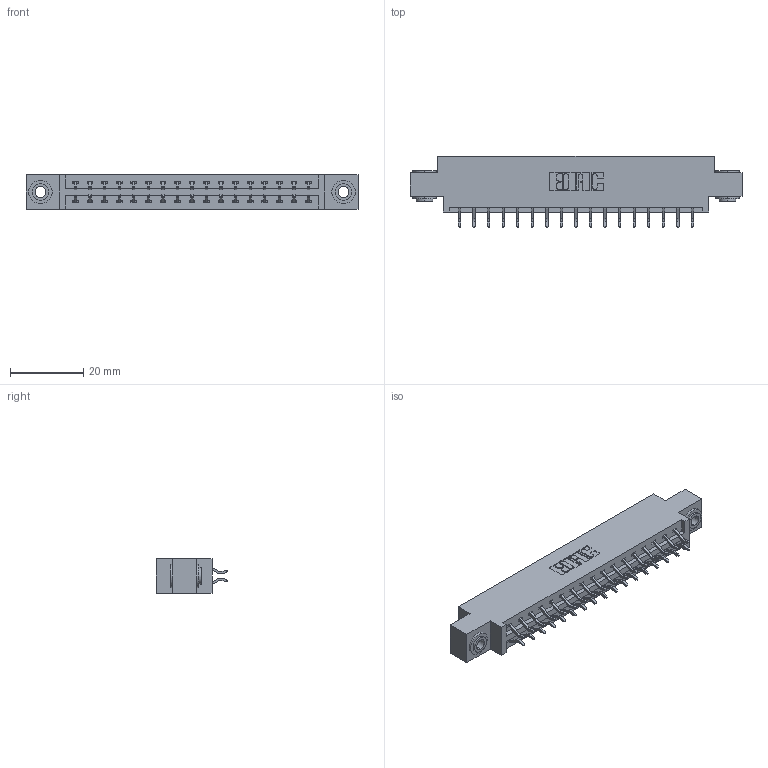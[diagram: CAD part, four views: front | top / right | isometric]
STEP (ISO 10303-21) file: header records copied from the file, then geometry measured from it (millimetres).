
FILE_DESCRIPTION (( 'STEP AP203' ), '1' );
FILE_NAME ('337-034-556-803.STEP', '2018-08-07T13:22:19', ( '' ), ( '' ), 'SwSTEP 2.0', 'SolidWorks 2016', '' );
FILE_SCHEMA (( 'CONFIG_CONTROL_DESIGN' ));
Length unit declared in the file: inch
Products named in the file (4): 345-292-001_556 Tail; 345-250-002_345-250-002-102; 337-034-556-803; 337 Part_0.170 Offset - 0.156 Dia-TH
Assembly tree (37 placements, depth 2):
  337-034-556-803
    337 Part_0.170 Offset - 0.156 Dia-TH
    345-292-001_556 Tail  x34
    345-250-002_345-250-002-102  x2
Bounding box: 90.37 x 19.57 x 9.4 mm (x, y, z)
Volume: 9092 mm3; surface area: 10332.1 mm2
Topology: 37 solids, 37 shells, 2196 faces, 6485 edges, 4274 vertices
Faces by surface type: plane 1512, cylinder 676, cone 8
Entity records: 17416 total; most frequent: CARTESIAN_POINT 2945, ORIENTED_EDGE 2862, DIRECTION 2573, EDGE_CURVE 1431, VECTOR 1271, LINE 1271, VERTEX_POINT 950, AXIS2_PLACEMENT_3D 651
